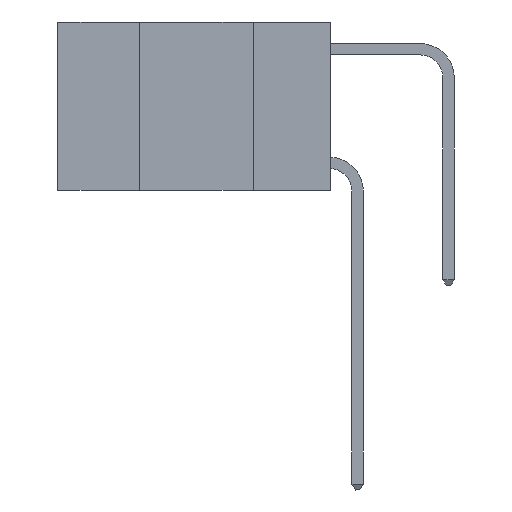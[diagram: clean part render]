
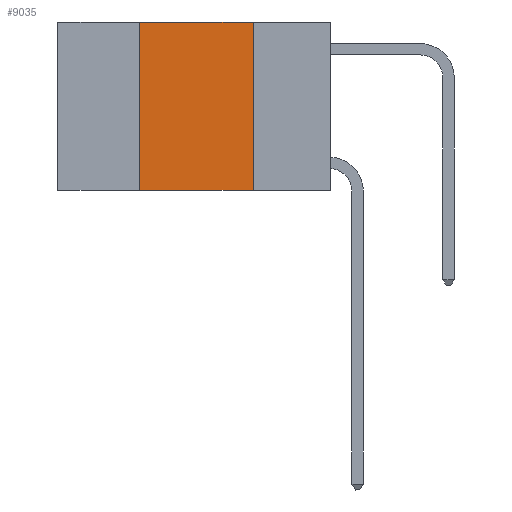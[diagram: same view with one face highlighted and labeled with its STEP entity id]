
A CAD part, left-side view. The second image highlights one B-rep face of the part: STEP entity #9035.
In plain terms, the highlighted planar face has unit normal (-1, 0, 0).
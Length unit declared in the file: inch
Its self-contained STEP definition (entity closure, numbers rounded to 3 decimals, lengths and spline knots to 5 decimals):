
#1174 = ORIENTED_EDGE ( 'NONE', *, *, #9951, .F. ) ;
#1803 = EDGE_LOOP ( 'NONE', ( #6981, #15103, #1174, #13594 ) ) ;
#2146 = VECTOR ( 'NONE', #10638, 39.37008 ) ;
#2238 = DIRECTION ( 'NONE',  ( 0., 0., -1. ) ) ;
#2832 = CARTESIAN_POINT ( 'NONE',  ( 0., 0.6, 0. ) ) ;
#5181 = EDGE_CURVE ( 'NONE', #8925, #11959, #16508, .T. ) ;
#5260 = CARTESIAN_POINT ( 'NONE',  ( 0., 0.42, 0. ) ) ;
#5395 = CARTESIAN_POINT ( 'NONE',  ( 0., 0.6, 0. ) ) ;
#6329 = CARTESIAN_POINT ( 'NONE',  ( 0., 0.42, 0. ) ) ;
#6981 = ORIENTED_EDGE ( 'NONE', *, *, #5181, .F. ) ;
#8220 = VERTEX_POINT ( 'NONE', #8381 ) ;
#8381 = CARTESIAN_POINT ( 'NONE',  ( 0., 0.42, -0.37 ) ) ;
#8925 = VERTEX_POINT ( 'NONE', #13680 ) ;
#8980 = DIRECTION ( 'NONE',  ( 0., 0., 1. ) ) ;
#9035 = ADVANCED_FACE ( 'NONE', ( #9539 ), #15771, .F. ) ;
#9264 = EDGE_CURVE ( 'NONE', #13799, #8925, #14564, .T. ) ;
#9539 = FACE_OUTER_BOUND ( 'NONE', #1803, .T. ) ;
#9951 = EDGE_CURVE ( 'NONE', #8220, #13799, #11805, .T. ) ;
#10159 = CARTESIAN_POINT ( 'NONE',  ( 0., 0.17, -0.37 ) ) ;
#10638 = DIRECTION ( 'NONE',  ( 0., -1., 0. ) ) ;
#10659 = DIRECTION ( 'NONE',  ( 1., 0., 0. ) ) ;
#10943 = CARTESIAN_POINT ( 'NONE',  ( 0., 0.6, -0.37 ) ) ;
#11023 = LINE ( 'NONE', #10943, #13766 ) ;
#11805 = LINE ( 'NONE', #5260, #13144 ) ;
#11959 = VERTEX_POINT ( 'NONE', #10159 ) ;
#12138 = DIRECTION ( 'NONE',  ( 0., 0., -1. ) ) ;
#12338 = DIRECTION ( 'NONE',  ( 0., -1., 0. ) ) ;
#13144 = VECTOR ( 'NONE', #8980, 39.37008 ) ;
#13536 = EDGE_CURVE ( 'NONE', #8220, #11959, #11023, .T. ) ;
#13594 = ORIENTED_EDGE ( 'NONE', *, *, #13536, .T. ) ;
#13680 = CARTESIAN_POINT ( 'NONE',  ( 0., 0.17, 0. ) ) ;
#13742 = VECTOR ( 'NONE', #2238, 39.37008 ) ;
#13766 = VECTOR ( 'NONE', #12338, 39.37008 ) ;
#13799 = VERTEX_POINT ( 'NONE', #6329 ) ;
#13982 = CARTESIAN_POINT ( 'NONE',  ( 0., 0.17, 0. ) ) ;
#14564 = LINE ( 'NONE', #2832, #2146 ) ;
#15103 = ORIENTED_EDGE ( 'NONE', *, *, #9264, .F. ) ;
#15771 = PLANE ( 'NONE',  #16923 ) ;
#16508 = LINE ( 'NONE', #13982, #13742 ) ;
#16923 = AXIS2_PLACEMENT_3D ( 'NONE', #5395, #10659, #12138 ) ;
